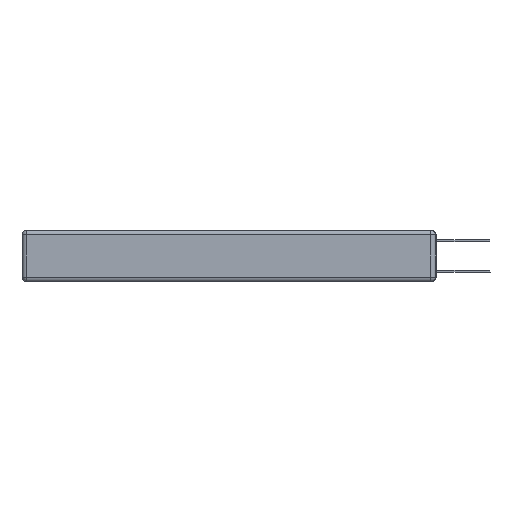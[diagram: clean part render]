
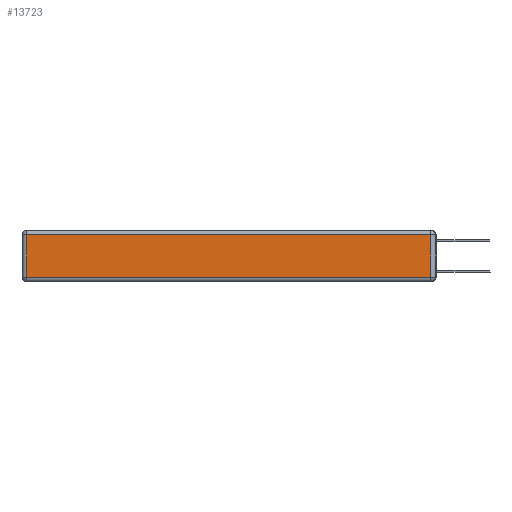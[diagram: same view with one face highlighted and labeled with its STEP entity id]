
A CAD part, left-side view. The second image highlights one B-rep face of the part: STEP entity #13723.
In plain terms, the highlighted planar face has unit normal (-1, 0, 0).
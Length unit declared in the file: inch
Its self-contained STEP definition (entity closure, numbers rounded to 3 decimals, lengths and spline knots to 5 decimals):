
#905 = VERTEX_POINT ( 'NONE', #1182 ) ;
#1182 = CARTESIAN_POINT ( 'NONE',  ( 0., 0.03, -0.03 ) ) ;
#1324 = FACE_OUTER_BOUND ( 'NONE', #9175, .T. ) ;
#1544 = LINE ( 'NONE', #5078, #10767 ) ;
#4675 = PLANE ( 'NONE',  #15802 ) ;
#4684 = LINE ( 'NONE', #17005, #4923 ) ;
#4819 = ORIENTED_EDGE ( 'NONE', *, *, #16611, .T. ) ;
#4923 = VECTOR ( 'NONE', #18845, 39.37008 ) ;
#5078 = CARTESIAN_POINT ( 'NONE',  ( 0., 2.75, -0.03 ) ) ;
#5132 = CARTESIAN_POINT ( 'NONE',  ( 0., 0.03, -0.313 ) ) ;
#6487 = DIRECTION ( 'NONE',  ( -1., 0., 0. ) ) ;
#7385 = CARTESIAN_POINT ( 'NONE',  ( 0., 2.72, -0.313 ) ) ;
#7794 = CARTESIAN_POINT ( 'NONE',  ( 0., 2.72, -0.03 ) ) ;
#8763 = VERTEX_POINT ( 'NONE', #7385 ) ;
#8871 = VECTOR ( 'NONE', #15843, 39.37008 ) ;
#9175 = EDGE_LOOP ( 'NONE', ( #19597, #11176, #4819, #17842 ) ) ;
#9936 = EDGE_CURVE ( 'NONE', #14985, #8763, #4684, .T. ) ;
#10377 = CARTESIAN_POINT ( 'NONE',  ( 0., 0.03, -0.343 ) ) ;
#10767 = VECTOR ( 'NONE', #20696, 39.37008 ) ;
#11176 = ORIENTED_EDGE ( 'NONE', *, *, #18686, .T. ) ;
#11454 = LINE ( 'NONE', #10377, #14190 ) ;
#13345 = DIRECTION ( 'NONE',  ( 0., 0., 1. ) ) ;
#13723 = ADVANCED_FACE ( 'NONE', ( #1324 ), #4675, .T. ) ;
#13895 = VERTEX_POINT ( 'NONE', #5132 ) ;
#14190 = VECTOR ( 'NONE', #19098, 39.37008 ) ;
#14753 = EDGE_CURVE ( 'NONE', #8763, #13895, #15914, .T. ) ;
#14985 = VERTEX_POINT ( 'NONE', #7794 ) ;
#15802 = AXIS2_PLACEMENT_3D ( 'NONE', #20153, #6487, #13345 ) ;
#15843 = DIRECTION ( 'NONE',  ( 0., -1., 0. ) ) ;
#15914 = LINE ( 'NONE', #19272, #8871 ) ;
#16611 = EDGE_CURVE ( 'NONE', #905, #14985, #1544, .T. ) ;
#17005 = CARTESIAN_POINT ( 'NONE',  ( 0., 2.72, -0.343 ) ) ;
#17842 = ORIENTED_EDGE ( 'NONE', *, *, #9936, .T. ) ;
#18686 = EDGE_CURVE ( 'NONE', #13895, #905, #11454, .T. ) ;
#18845 = DIRECTION ( 'NONE',  ( 0., 0., -1. ) ) ;
#19098 = DIRECTION ( 'NONE',  ( 0., 0., 1. ) ) ;
#19272 = CARTESIAN_POINT ( 'NONE',  ( 0., 0., -0.313 ) ) ;
#19597 = ORIENTED_EDGE ( 'NONE', *, *, #14753, .T. ) ;
#20153 = CARTESIAN_POINT ( 'NONE',  ( 0., 0., -0.343 ) ) ;
#20696 = DIRECTION ( 'NONE',  ( 0., 1., 0. ) ) ;
